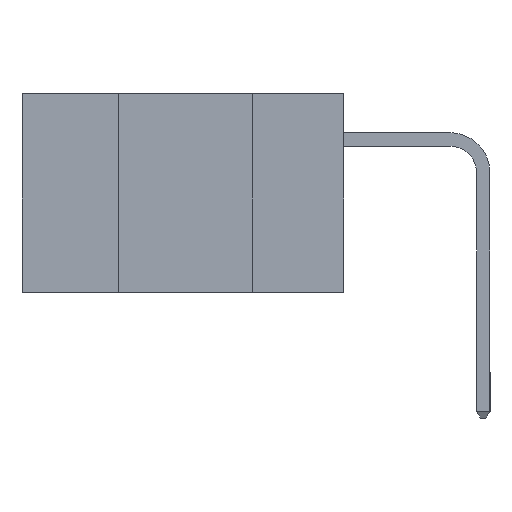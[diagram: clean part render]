
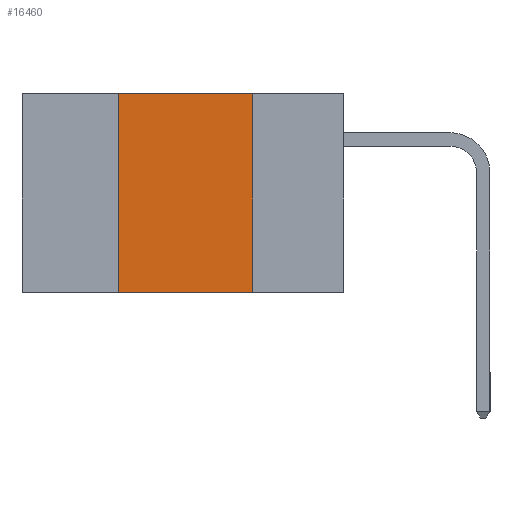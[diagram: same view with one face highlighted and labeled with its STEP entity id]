
A CAD part, left-side view. The second image highlights one B-rep face of the part: STEP entity #16460.
In plain terms, the highlighted planar face has unit normal (-1, 0, 0).
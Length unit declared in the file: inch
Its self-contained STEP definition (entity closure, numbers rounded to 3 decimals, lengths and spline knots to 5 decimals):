
#12 = LINE ( 'NONE', #3218, #6739 ) ;
#193 = CARTESIAN_POINT ( 'NONE',  ( 0., 0.42, 0. ) ) ;
#1501 = EDGE_CURVE ( 'NONE', #13051, #16219, #2796, .T. ) ;
#1594 = VECTOR ( 'NONE', #3063, 39.37008 ) ;
#1668 = DIRECTION ( 'NONE',  ( 0., 0., -1. ) ) ;
#1944 = CARTESIAN_POINT ( 'NONE',  ( 0., 0.17, -0.37 ) ) ;
#2298 = CARTESIAN_POINT ( 'NONE',  ( 0., 0.42, -0.37 ) ) ;
#2579 = CARTESIAN_POINT ( 'NONE',  ( 0., 0.6, 0. ) ) ;
#2796 = LINE ( 'NONE', #2579, #7333 ) ;
#3063 = DIRECTION ( 'NONE',  ( 0., 0., 1. ) ) ;
#3218 = CARTESIAN_POINT ( 'NONE',  ( 0., 0.17, 0. ) ) ;
#3386 = DIRECTION ( 'NONE',  ( 1., 0., 0. ) ) ;
#3453 = PLANE ( 'NONE',  #14672 ) ;
#5219 = ORIENTED_EDGE ( 'NONE', *, *, #1501, .F. ) ;
#5675 = CARTESIAN_POINT ( 'NONE',  ( 0., 0.17, 0. ) ) ;
#6739 = VECTOR ( 'NONE', #1668, 39.37008 ) ;
#7333 = VECTOR ( 'NONE', #17844, 39.37008 ) ;
#8512 = CARTESIAN_POINT ( 'NONE',  ( 0., 0.42, 0. ) ) ;
#9347 = FACE_OUTER_BOUND ( 'NONE', #12644, .T. ) ;
#9596 = ORIENTED_EDGE ( 'NONE', *, *, #11132, .T. ) ;
#9744 = VERTEX_POINT ( 'NONE', #1944 ) ;
#11132 = EDGE_CURVE ( 'NONE', #12141, #9744, #18150, .T. ) ;
#12141 = VERTEX_POINT ( 'NONE', #2298 ) ;
#12232 = ORIENTED_EDGE ( 'NONE', *, *, #19239, .F. ) ;
#12370 = CARTESIAN_POINT ( 'NONE',  ( 0., 0.6, -0.37 ) ) ;
#12644 = EDGE_LOOP ( 'NONE', ( #17252, #5219, #12232, #9596 ) ) ;
#13051 = VERTEX_POINT ( 'NONE', #8512 ) ;
#13531 = LINE ( 'NONE', #193, #1594 ) ;
#13924 = DIRECTION ( 'NONE',  ( 0., 0., -1. ) ) ;
#14122 = CARTESIAN_POINT ( 'NONE',  ( 0., 0.6, 0. ) ) ;
#14672 = AXIS2_PLACEMENT_3D ( 'NONE', #14122, #3386, #13924 ) ;
#15300 = DIRECTION ( 'NONE',  ( 0., -1., 0. ) ) ;
#16219 = VERTEX_POINT ( 'NONE', #5675 ) ;
#16416 = EDGE_CURVE ( 'NONE', #16219, #9744, #12, .T. ) ;
#16460 = ADVANCED_FACE ( 'NONE', ( #9347 ), #3453, .F. ) ;
#17252 = ORIENTED_EDGE ( 'NONE', *, *, #16416, .F. ) ;
#17844 = DIRECTION ( 'NONE',  ( 0., -1., 0. ) ) ;
#18150 = LINE ( 'NONE', #12370, #19298 ) ;
#19239 = EDGE_CURVE ( 'NONE', #12141, #13051, #13531, .T. ) ;
#19298 = VECTOR ( 'NONE', #15300, 39.37008 ) ;
